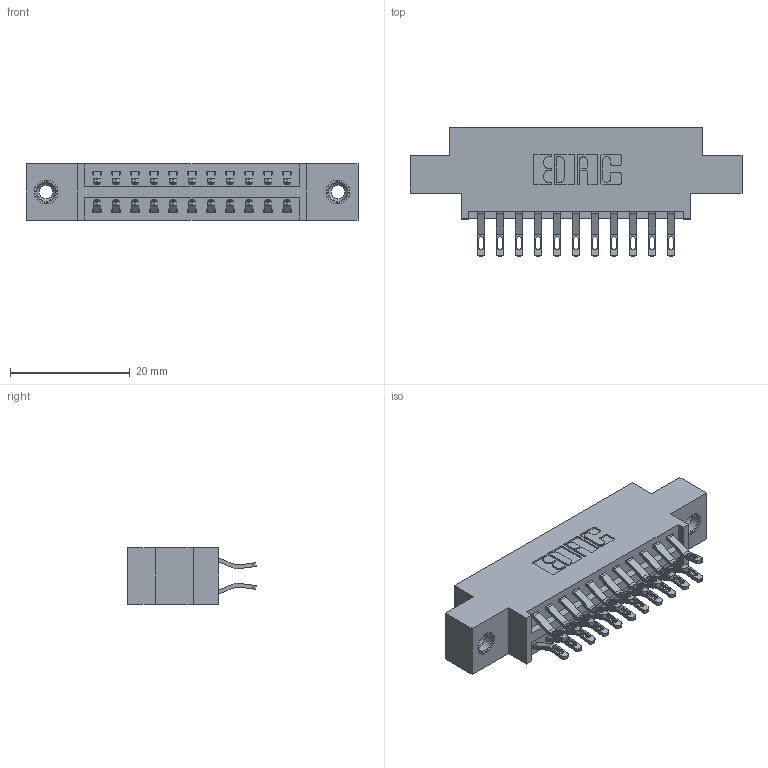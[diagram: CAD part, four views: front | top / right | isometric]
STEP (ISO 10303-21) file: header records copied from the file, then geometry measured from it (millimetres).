
FILE_DESCRIPTION (( 'STEP AP203' ), '1' );
FILE_NAME ('396-022-555-808.STEP', '2019-11-01T18:32:29', ( '' ), ( '' ), 'SwSTEP 2.0', 'SolidWorks 2016', '' );
FILE_SCHEMA (( 'CONFIG_CONTROL_DESIGN' ));
Length unit declared in the file: inch
Products named in the file (4): 346 Part_0.170 Offset - 0.156 Dia-TI; 345-292-001_555 Tail; 345-250-001_345-250-003-102; 396-022-555-808
Assembly tree (25 placements, depth 2):
  396-022-555-808
    346 Part_0.170 Offset - 0.156 Dia-TI
    345-292-001_555 Tail  x22
    345-250-001_345-250-003-102  x2
Bounding box: 55.5 x 21.46 x 9.4 mm (x, y, z)
Volume: 5073.8 mm3; surface area: 6914.1 mm2
Topology: 25 solids, 25 shells, 1462 faces, 4503 edges, 2994 vertices
Faces by surface type: plane 838, cylinder 608, cone 12, torus 4
Entity records: 12996 total; most frequent: CARTESIAN_POINT 2205, ORIENTED_EDGE 2102, DIRECTION 1989, EDGE_CURVE 1051, LINE 835, VECTOR 835, VERTEX_POINT 696, AXIS2_PLACEMENT_3D 577
